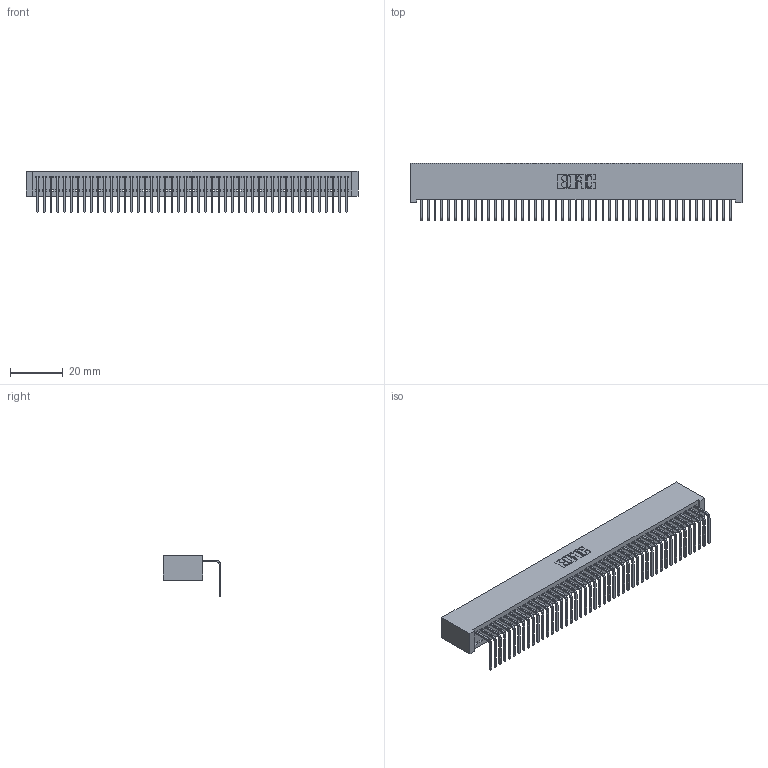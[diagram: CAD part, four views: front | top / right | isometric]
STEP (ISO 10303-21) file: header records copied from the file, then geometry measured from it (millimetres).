
FILE_DESCRIPTION (( 'STEP AP203' ), '1' );
FILE_NAME ('392-047-558-101.STEP', '2019-10-08T00:33:44', ( '' ), ( '' ), 'SwSTEP 2.0', 'SolidWorks 2016', '' );
FILE_SCHEMA (( 'CONFIG_CONTROL_DESIGN' ));
Length unit declared in the file: inch
Products named in the file (3): 342 Part_Lugless; 345-292-001_558 Tail - 2; 392-047-558-101
Assembly tree (48 placements, depth 2):
  392-047-558-101
    342 Part_Lugless
    345-292-001_558 Tail - 2  x47
Bounding box: 125.63 x 21.91 x 15.62 mm (x, y, z)
Volume: 11599.1 mm3; surface area: 18338.7 mm2
Topology: 48 solids, 48 shells, 2922 faces, 8829 edges, 5822 vertices
Faces by surface type: plane 2130, cylinder 792
Entity records: 27761 total; most frequent: CARTESIAN_POINT 4795, ORIENTED_EDGE 4778, DIRECTION 4027, EDGE_CURVE 2389, LINE 2269, VECTOR 2269, VERTEX_POINT 1590, AXIS2_PLACEMENT_3D 879
